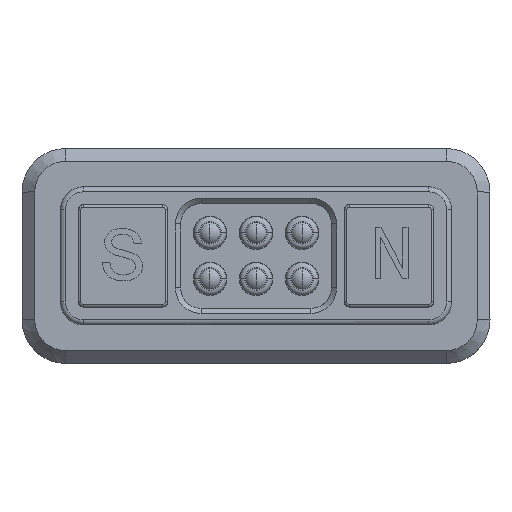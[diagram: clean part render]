
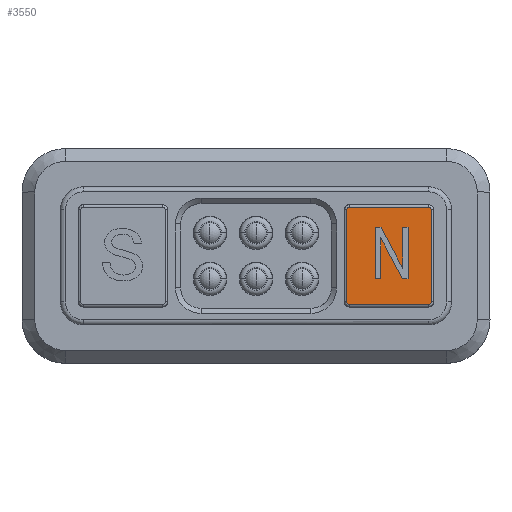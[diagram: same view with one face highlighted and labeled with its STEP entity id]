
A CAD part, top view. The second image highlights one B-rep face of the part: STEP entity #3550.
In plain terms, the highlighted planar face has unit normal (0, 0, 1).
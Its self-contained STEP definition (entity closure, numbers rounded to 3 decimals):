
#5 = EDGE_CURVE ( 'NONE', #455, #10765, #11279, .T. ) ;
#63 = VERTEX_POINT ( 'NONE', #16490 ) ;
#93 = LINE ( 'NONE', #18158, #15913 ) ;
#148 = CARTESIAN_POINT ( 'NONE',  ( 4.879, 0.704, 4.5 ) ) ;
#170 = VECTOR ( 'NONE', #15035, 1000. ) ;
#285 = DIRECTION ( 'NONE',  ( 1., 0., 0. ) ) ;
#369 = VECTOR ( 'NONE', #20069, 1000. ) ;
#455 = VERTEX_POINT ( 'NONE', #4928 ) ;
#666 = CARTESIAN_POINT ( 'NONE',  ( 3.65, -1.9, 4.5 ) ) ;
#949 = VECTOR ( 'NONE', #14071, 1000. ) ;
#1414 = ORIENTED_EDGE ( 'NONE', *, *, #15695, .T. ) ;
#1424 = ORIENTED_EDGE ( 'NONE', *, *, #2399, .T. ) ;
#1434 = DIRECTION ( 'NONE',  ( 0., 1., 0. ) ) ;
#1520 = CARTESIAN_POINT ( 'NONE',  ( 3.55, 1.8, 4.5 ) ) ;
#1864 = CARTESIAN_POINT ( 'NONE',  ( 6.75, 1.9, 4.5 ) ) ;
#1880 = EDGE_CURVE ( 'NONE', #13165, #18133, #4593, .T. ) ;
#2196 = LINE ( 'NONE', #15256, #369 ) ;
#2399 = EDGE_CURVE ( 'NONE', #4950, #16243, #2196, .T. ) ;
#2617 = DIRECTION ( 'NONE',  ( 0., 0., 1. ) ) ;
#2721 = CARTESIAN_POINT ( 'NONE',  ( 3.55, -1.8, 4.5 ) ) ;
#2729 = EDGE_LOOP ( 'NONE', ( #11501, #1424, #19249, #12940, #9586, #12164, #1414, #14444, #8133, #13830 ) ) ;
#2809 = VERTEX_POINT ( 'NONE', #8608 ) ;
#2870 = EDGE_CURVE ( 'NONE', #16581, #10965, #8824, .T. ) ;
#2998 = VECTOR ( 'NONE', #12168, 1000. ) ;
#3081 = VECTOR ( 'NONE', #14641, 1000. ) ;
#3171 = EDGE_CURVE ( 'NONE', #18448, #3706, #8666, .T. ) ;
#3269 = ORIENTED_EDGE ( 'NONE', *, *, #21088, .T. ) ;
#3365 = CARTESIAN_POINT ( 'NONE',  ( 6.75, -1.8, 4.5 ) ) ;
#3550 = ADVANCED_FACE ( 'NONE', ( #8747, #16869 ), #17075, .T. ) ;
#3706 = VERTEX_POINT ( 'NONE', #2721 ) ;
#3749 = ORIENTED_EDGE ( 'NONE', *, *, #5375, .T. ) ;
#4415 = VECTOR ( 'NONE', #4985, 1000. ) ;
#4511 = VERTEX_POINT ( 'NONE', #13092 ) ;
#4552 = LINE ( 'NONE', #4981, #15814 ) ;
#4571 = VECTOR ( 'NONE', #10482, 1000. ) ;
#4593 = LINE ( 'NONE', #8119, #3081 ) ;
#4623 = EDGE_CURVE ( 'NONE', #3706, #5355, #11015, .T. ) ;
#4928 = CARTESIAN_POINT ( 'NONE',  ( 5.721, -0.888, 4.5 ) ) ;
#4950 = VERTEX_POINT ( 'NONE', #18263 ) ;
#4959 = CARTESIAN_POINT ( 'NONE',  ( 6.75, 1.8, 4.5 ) ) ;
#4981 = CARTESIAN_POINT ( 'NONE',  ( 5.944, -0.888, 4.5 ) ) ;
#4985 = DIRECTION ( 'NONE',  ( 0., 1., 0. ) ) ;
#5103 = LINE ( 'NONE', #14934, #6995 ) ;
#5285 = EDGE_CURVE ( 'NONE', #10965, #455, #4552, .T. ) ;
#5355 = VERTEX_POINT ( 'NONE', #666 ) ;
#5375 = EDGE_CURVE ( 'NONE', #2809, #63, #7295, .T. ) ;
#5624 = CARTESIAN_POINT ( 'NONE',  ( 4.671, -0.888, 4.5 ) ) ;
#5651 = CARTESIAN_POINT ( 'NONE',  ( 6.85, -1.8, 4.5 ) ) ;
#5673 = EDGE_CURVE ( 'NONE', #16243, #15265, #6953, .T. ) ;
#5799 = CARTESIAN_POINT ( 'NONE',  ( 3.55, 1.8, 4.5 ) ) ;
#6288 = VECTOR ( 'NONE', #9033, 1000. ) ;
#6641 = CARTESIAN_POINT ( 'NONE',  ( 6.75, -1.9, 4.5 ) ) ;
#6953 = LINE ( 'NONE', #8782, #4571 ) ;
#6995 = VECTOR ( 'NONE', #285, 1000. ) ;
#7033 = LINE ( 'NONE', #5651, #2998 ) ;
#7295 = LINE ( 'NONE', #1864, #9344 ) ;
#7411 = CARTESIAN_POINT ( 'NONE',  ( 5.944, 1.112, 4.5 ) ) ;
#7596 = VERTEX_POINT ( 'NONE', #14861 ) ;
#7619 = VERTEX_POINT ( 'NONE', #8670 ) ;
#8119 = CARTESIAN_POINT ( 'NONE',  ( 4.892, 1.112, 4.5 ) ) ;
#8133 = ORIENTED_EDGE ( 'NONE', *, *, #5285, .T. ) ;
#8372 = EDGE_CURVE ( 'NONE', #11132, #7596, #19574, .T. ) ;
#8403 = DIRECTION ( 'NONE',  ( -1., 0., 0. ) ) ;
#8584 = CIRCLE ( 'NONE', #14044, 0.1 ) ;
#8608 = CARTESIAN_POINT ( 'NONE',  ( 6.75, 1.9, 4.5 ) ) ;
#8651 = DIRECTION ( 'NONE',  ( 1., 0., 0. ) ) ;
#8666 = LINE ( 'NONE', #1520, #17218 ) ;
#8670 = CARTESIAN_POINT ( 'NONE',  ( 5.736, 1.112, 4.5 ) ) ;
#8747 = FACE_OUTER_BOUND ( 'NONE', #10153, .T. ) ;
#8782 = CARTESIAN_POINT ( 'NONE',  ( 4.671, -0.888, 4.5 ) ) ;
#8824 = LINE ( 'NONE', #7411, #6288 ) ;
#8888 = ORIENTED_EDGE ( 'NONE', *, *, #18604, .T. ) ;
#9029 = DIRECTION ( 'NONE',  ( -1., 0., 0. ) ) ;
#9033 = DIRECTION ( 'NONE',  ( 0., -1., 0. ) ) ;
#9344 = VECTOR ( 'NONE', #8403, 1000. ) ;
#9586 = ORIENTED_EDGE ( 'NONE', *, *, #1880, .T. ) ;
#9780 = DIRECTION ( 'NONE',  ( 0., 0., 1. ) ) ;
#9892 = DIRECTION ( 'NONE',  ( 0., 0., 1. ) ) ;
#10153 = EDGE_LOOP ( 'NONE', ( #20148, #16336, #8888, #12860, #3749, #3269, #20103, #18888 ) ) ;
#10186 = DIRECTION ( 'NONE',  ( 0., 0., 1. ) ) ;
#10435 = LINE ( 'NONE', #16969, #949 ) ;
#10482 = DIRECTION ( 'NONE',  ( 0., 1., 0. ) ) ;
#10737 = CARTESIAN_POINT ( 'NONE',  ( 5.944, 1.112, 4.5 ) ) ;
#10765 = VERTEX_POINT ( 'NONE', #148 ) ;
#10965 = VERTEX_POINT ( 'NONE', #16939 ) ;
#11015 = CIRCLE ( 'NONE', #15110, 0.1 ) ;
#11132 = VERTEX_POINT ( 'NONE', #6641 ) ;
#11279 = LINE ( 'NONE', #19080, #14393 ) ;
#11501 = ORIENTED_EDGE ( 'NONE', *, *, #18106, .T. ) ;
#12164 = ORIENTED_EDGE ( 'NONE', *, *, #12577, .T. ) ;
#12168 = DIRECTION ( 'NONE',  ( 0., 1., 0. ) ) ;
#12184 = EDGE_CURVE ( 'NONE', #5355, #11132, #93, .T. ) ;
#12432 = CARTESIAN_POINT ( 'NONE',  ( 3.65, -1.8, 4.5 ) ) ;
#12577 = EDGE_CURVE ( 'NONE', #18133, #7619, #19638, .T. ) ;
#12798 = AXIS2_PLACEMENT_3D ( 'NONE', #15564, #2617, #15667 ) ;
#12860 = ORIENTED_EDGE ( 'NONE', *, *, #12994, .T. ) ;
#12940 = ORIENTED_EDGE ( 'NONE', *, *, #15708, .T. ) ;
#12994 = EDGE_CURVE ( 'NONE', #4511, #2809, #17746, .T. ) ;
#13092 = CARTESIAN_POINT ( 'NONE',  ( 6.85, 1.8, 4.5 ) ) ;
#13165 = VERTEX_POINT ( 'NONE', #20549 ) ;
#13323 = LINE ( 'NONE', #18028, #170 ) ;
#13425 = CARTESIAN_POINT ( 'NONE',  ( 5.736, -0.483, 4.5 ) ) ;
#13664 = AXIS2_PLACEMENT_3D ( 'NONE', #4959, #10186, #16716 ) ;
#13830 = ORIENTED_EDGE ( 'NONE', *, *, #5, .T. ) ;
#14044 = AXIS2_PLACEMENT_3D ( 'NONE', #14701, #9780, #1434 ) ;
#14071 = DIRECTION ( 'NONE',  ( 0., -1., 0. ) ) ;
#14393 = VECTOR ( 'NONE', #17795, 1000. ) ;
#14444 = ORIENTED_EDGE ( 'NONE', *, *, #2870, .T. ) ;
#14641 = DIRECTION ( 'NONE',  ( 0.468, -0.884, 0. ) ) ;
#14701 = CARTESIAN_POINT ( 'NONE',  ( 3.65, 1.8, 4.5 ) ) ;
#14851 = CARTESIAN_POINT ( 'NONE',  ( 4.671, 1.112, 4.5 ) ) ;
#14861 = CARTESIAN_POINT ( 'NONE',  ( 6.85, -1.8, 4.5 ) ) ;
#14934 = CARTESIAN_POINT ( 'NONE',  ( 4.671, 1.112, 4.5 ) ) ;
#15035 = DIRECTION ( 'NONE',  ( 1., 0., 0. ) ) ;
#15110 = AXIS2_PLACEMENT_3D ( 'NONE', #12432, #18748, #9029 ) ;
#15256 = CARTESIAN_POINT ( 'NONE',  ( 4.879, -0.888, 4.5 ) ) ;
#15265 = VERTEX_POINT ( 'NONE', #14851 ) ;
#15337 = DIRECTION ( 'NONE',  ( 0., -1., 0. ) ) ;
#15358 = CARTESIAN_POINT ( 'NONE',  ( 5.736, -0.483, 4.5 ) ) ;
#15564 = CARTESIAN_POINT ( 'NONE',  ( 5.2, 0., 4.5 ) ) ;
#15667 = DIRECTION ( 'NONE',  ( 1., 0., 0. ) ) ;
#15691 = DIRECTION ( 'NONE',  ( 0., -1., 0. ) ) ;
#15695 = EDGE_CURVE ( 'NONE', #7619, #16581, #13323, .T. ) ;
#15708 = EDGE_CURVE ( 'NONE', #15265, #13165, #5103, .T. ) ;
#15814 = VECTOR ( 'NONE', #16099, 1000. ) ;
#15913 = VECTOR ( 'NONE', #8651, 1000. ) ;
#16099 = DIRECTION ( 'NONE',  ( -1., 0., 0. ) ) ;
#16243 = VERTEX_POINT ( 'NONE', #5624 ) ;
#16336 = ORIENTED_EDGE ( 'NONE', *, *, #8372, .T. ) ;
#16490 = CARTESIAN_POINT ( 'NONE',  ( 3.65, 1.9, 4.5 ) ) ;
#16581 = VERTEX_POINT ( 'NONE', #10737 ) ;
#16716 = DIRECTION ( 'NONE',  ( 1., 0., 0. ) ) ;
#16869 = FACE_BOUND ( 'NONE', #2729, .T. ) ;
#16939 = CARTESIAN_POINT ( 'NONE',  ( 5.944, -0.888, 4.5 ) ) ;
#16969 = CARTESIAN_POINT ( 'NONE',  ( 4.879, 0.704, 4.5 ) ) ;
#17075 = PLANE ( 'NONE',  #12798 ) ;
#17218 = VECTOR ( 'NONE', #15691, 1000. ) ;
#17746 = CIRCLE ( 'NONE', #13664, 0.1 ) ;
#17795 = DIRECTION ( 'NONE',  ( -0.468, 0.884, 0. ) ) ;
#18028 = CARTESIAN_POINT ( 'NONE',  ( 5.736, 1.112, 4.5 ) ) ;
#18106 = EDGE_CURVE ( 'NONE', #10765, #4950, #10435, .T. ) ;
#18133 = VERTEX_POINT ( 'NONE', #15358 ) ;
#18158 = CARTESIAN_POINT ( 'NONE',  ( 3.65, -1.9, 4.5 ) ) ;
#18191 = AXIS2_PLACEMENT_3D ( 'NONE', #3365, #9892, #15337 ) ;
#18263 = CARTESIAN_POINT ( 'NONE',  ( 4.879, -0.888, 4.5 ) ) ;
#18448 = VERTEX_POINT ( 'NONE', #5799 ) ;
#18604 = EDGE_CURVE ( 'NONE', #7596, #4511, #7033, .T. ) ;
#18748 = DIRECTION ( 'NONE',  ( 0., 0., 1. ) ) ;
#18888 = ORIENTED_EDGE ( 'NONE', *, *, #4623, .T. ) ;
#19080 = CARTESIAN_POINT ( 'NONE',  ( 5.721, -0.888, 4.5 ) ) ;
#19249 = ORIENTED_EDGE ( 'NONE', *, *, #5673, .T. ) ;
#19574 = CIRCLE ( 'NONE', #18191, 0.1 ) ;
#19638 = LINE ( 'NONE', #13425, #4415 ) ;
#20069 = DIRECTION ( 'NONE',  ( -1., 0., 0. ) ) ;
#20103 = ORIENTED_EDGE ( 'NONE', *, *, #3171, .T. ) ;
#20148 = ORIENTED_EDGE ( 'NONE', *, *, #12184, .T. ) ;
#20549 = CARTESIAN_POINT ( 'NONE',  ( 4.892, 1.112, 4.5 ) ) ;
#21088 = EDGE_CURVE ( 'NONE', #63, #18448, #8584, .T. ) ;
